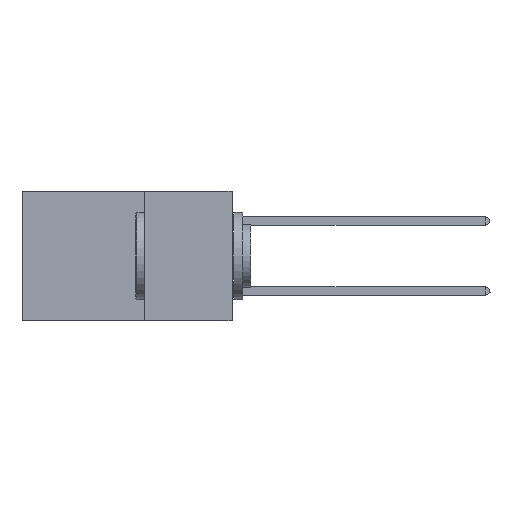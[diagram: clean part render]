
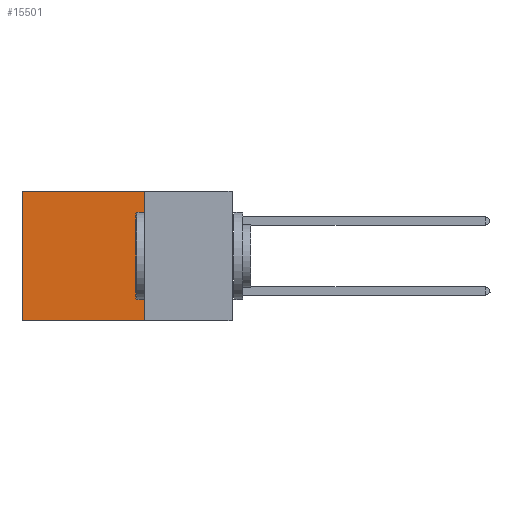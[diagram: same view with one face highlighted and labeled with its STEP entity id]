
A CAD part, left-side view. The second image highlights one B-rep face of the part: STEP entity #15501.
In plain terms, the highlighted planar face has unit normal (-1, 0, 0).
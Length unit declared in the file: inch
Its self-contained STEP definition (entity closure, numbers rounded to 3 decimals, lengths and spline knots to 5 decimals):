
#748 = ORIENTED_EDGE ( 'NONE', *, *, #3281, .F. ) ;
#1161 = DIRECTION ( 'NONE',  ( 0., 1., 0. ) ) ;
#1353 = CARTESIAN_POINT ( 'NONE',  ( 0.2875, 0.25, -0.37 ) ) ;
#1971 = CARTESIAN_POINT ( 'NONE',  ( 0.2875, 0.25, 0. ) ) ;
#2080 = AXIS2_PLACEMENT_3D ( 'NONE', #23827, #9011, #23914 ) ;
#3281 = EDGE_CURVE ( 'NONE', #10144, #20588, #23831, .T. ) ;
#3341 = EDGE_CURVE ( 'NONE', #11567, #23053, #15709, .T. ) ;
#6490 = EDGE_CURVE ( 'NONE', #23053, #20588, #6652, .T. ) ;
#6652 = LINE ( 'NONE', #18490, #22616 ) ;
#9011 = DIRECTION ( 'NONE',  ( 1., 0., 0. ) ) ;
#9606 = CARTESIAN_POINT ( 'NONE',  ( 0.2875, 0.25, 0. ) ) ;
#10144 = VERTEX_POINT ( 'NONE', #18690 ) ;
#10146 = VECTOR ( 'NONE', #26392, 39.37008 ) ;
#10792 = VECTOR ( 'NONE', #1161, 39.37008 ) ;
#11567 = VERTEX_POINT ( 'NONE', #1971 ) ;
#12536 = ORIENTED_EDGE ( 'NONE', *, *, #6490, .T. ) ;
#14320 = DIRECTION ( 'NONE',  ( 0., 0., -1. ) ) ;
#15087 = EDGE_CURVE ( 'NONE', #11567, #10144, #26145, .T. ) ;
#15402 = ORIENTED_EDGE ( 'NONE', *, *, #15087, .F. ) ;
#15501 = ADVANCED_FACE ( 'NONE', ( #23561 ), #21645, .F. ) ;
#15709 = LINE ( 'NONE', #9606, #10146 ) ;
#18490 = CARTESIAN_POINT ( 'NONE',  ( 0.2875, 0.6, 0. ) ) ;
#18690 = CARTESIAN_POINT ( 'NONE',  ( 0.2875, 0.25, -0.37 ) ) ;
#20588 = VERTEX_POINT ( 'NONE', #25647 ) ;
#20669 = VECTOR ( 'NONE', #23513, 39.37008 ) ;
#21079 = CARTESIAN_POINT ( 'NONE',  ( 0.2875, 0.25, 0. ) ) ;
#21645 = PLANE ( 'NONE',  #2080 ) ;
#22177 = CARTESIAN_POINT ( 'NONE',  ( 0.2875, 0.6, 0. ) ) ;
#22616 = VECTOR ( 'NONE', #14320, 39.37008 ) ;
#23053 = VERTEX_POINT ( 'NONE', #22177 ) ;
#23513 = DIRECTION ( 'NONE',  ( 0., 0., -1. ) ) ;
#23561 = FACE_OUTER_BOUND ( 'NONE', #23974, .T. ) ;
#23827 = CARTESIAN_POINT ( 'NONE',  ( 0.2875, 0.25, 0. ) ) ;
#23831 = LINE ( 'NONE', #1353, #10792 ) ;
#23914 = DIRECTION ( 'NONE',  ( 0., 0., -1. ) ) ;
#23974 = EDGE_LOOP ( 'NONE', ( #12536, #748, #15402, #25480 ) ) ;
#25480 = ORIENTED_EDGE ( 'NONE', *, *, #3341, .T. ) ;
#25647 = CARTESIAN_POINT ( 'NONE',  ( 0.2875, 0.6, -0.37 ) ) ;
#26145 = LINE ( 'NONE', #21079, #20669 ) ;
#26392 = DIRECTION ( 'NONE',  ( 0., 1., 0. ) ) ;
